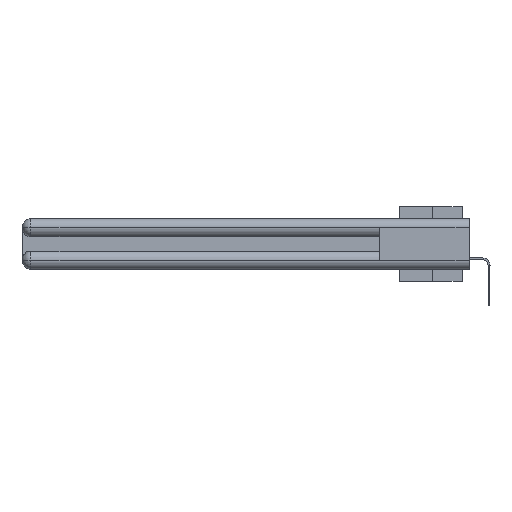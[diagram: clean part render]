
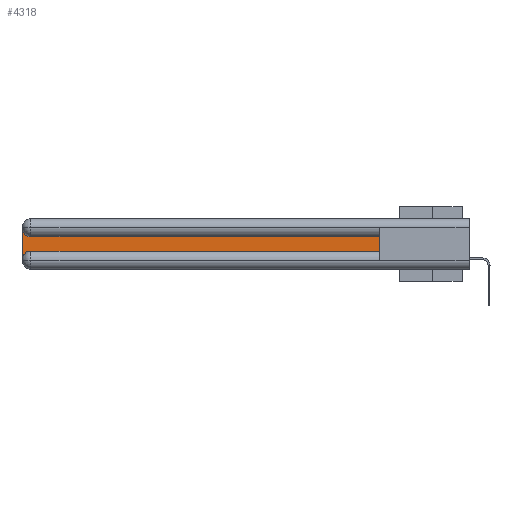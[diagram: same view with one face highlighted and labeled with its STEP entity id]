
A CAD part, left-side view. The second image highlights one B-rep face of the part: STEP entity #4318.
In plain terms, the highlighted planar face has unit normal (-1, 0, 0).
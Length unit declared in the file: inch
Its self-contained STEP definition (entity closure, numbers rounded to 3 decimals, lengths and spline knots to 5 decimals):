
#374 = CARTESIAN_POINT ( 'NONE',  ( 0.075, 2.94, -0.2775 ) ) ;
#1559 = LINE ( 'NONE', #11596, #24835 ) ;
#1977 = DIRECTION ( 'NONE',  ( 1., 0., 0. ) ) ;
#3443 = ORIENTED_EDGE ( 'NONE', *, *, #23956, .T. ) ;
#3686 = LINE ( 'NONE', #26589, #24172 ) ;
#4118 = VERTEX_POINT ( 'NONE', #25696 ) ;
#4223 = DIRECTION ( 'NONE',  ( 0., 0., -1. ) ) ;
#4318 = ADVANCED_FACE ( 'NONE', ( #4321 ), #12756, .F. ) ;
#4321 = FACE_OUTER_BOUND ( 'NONE', #5259, .T. ) ;
#4805 = DIRECTION ( 'NONE',  ( 1., 0., 0. ) ) ;
#5259 = EDGE_LOOP ( 'NONE', ( #17833, #15234, #28649, #16277, #9049, #3443 ) ) ;
#6048 = VERTEX_POINT ( 'NONE', #11331 ) ;
#7652 = VERTEX_POINT ( 'NONE', #13058 ) ;
#7880 = EDGE_CURVE ( 'NONE', #4118, #22042, #20739, .T. ) ;
#8345 = EDGE_CURVE ( 'NONE', #16306, #23847, #21772, .T. ) ;
#8831 = CARTESIAN_POINT ( 'NONE',  ( 0.075, 0.6, -0.2175 ) ) ;
#9049 = ORIENTED_EDGE ( 'NONE', *, *, #7880, .T. ) ;
#9163 = DIRECTION ( 'NONE',  ( 0., 0., -1. ) ) ;
#11331 = CARTESIAN_POINT ( 'NONE',  ( 0.075, 3., -0.2775 ) ) ;
#11596 = CARTESIAN_POINT ( 'NONE',  ( 0.075, 3., -0.2175 ) ) ;
#12555 = CARTESIAN_POINT ( 'NONE',  ( 0.075, 0.6, -0.2175 ) ) ;
#12756 = PLANE ( 'NONE',  #29003 ) ;
#13058 = CARTESIAN_POINT ( 'NONE',  ( 0.075, 0.6, -0.1225 ) ) ;
#13113 = CARTESIAN_POINT ( 'NONE',  ( 0.075, 2.94, -0.1225 ) ) ;
#13281 = CARTESIAN_POINT ( 'NONE',  ( 0.075, 2.94, -0.0625 ) ) ;
#14448 = DIRECTION ( 'NONE',  ( 0., -1., 0. ) ) ;
#14471 = DIRECTION ( 'NONE',  ( 0., 0., 1. ) ) ;
#15234 = ORIENTED_EDGE ( 'NONE', *, *, #8345, .T. ) ;
#15367 = EDGE_CURVE ( 'NONE', #6048, #4118, #16009, .T. ) ;
#16009 = CIRCLE ( 'NONE', #22250, 0.06 ) ;
#16148 = DIRECTION ( 'NONE',  ( 0., 0., -1. ) ) ;
#16277 = ORIENTED_EDGE ( 'NONE', *, *, #15367, .T. ) ;
#16306 = VERTEX_POINT ( 'NONE', #13113 ) ;
#16460 = AXIS2_PLACEMENT_3D ( 'NONE', #13281, #1977, #4223 ) ;
#16952 = CARTESIAN_POINT ( 'NONE',  ( 0.075, 0.6, -0.2175 ) ) ;
#17033 = DIRECTION ( 'NONE',  ( 0., 0., -1. ) ) ;
#17833 = ORIENTED_EDGE ( 'NONE', *, *, #27393, .T. ) ;
#19116 = EDGE_CURVE ( 'NONE', #23847, #6048, #1559, .T. ) ;
#20739 = LINE ( 'NONE', #12555, #27429 ) ;
#21772 = CIRCLE ( 'NONE', #16460, 0.06 ) ;
#21840 = CARTESIAN_POINT ( 'NONE',  ( 0.075, 3., -0.1225 ) ) ;
#22042 = VERTEX_POINT ( 'NONE', #8831 ) ;
#22250 = AXIS2_PLACEMENT_3D ( 'NONE', #374, #4805, #16148 ) ;
#22340 = DIRECTION ( 'NONE',  ( 0., 1., 0. ) ) ;
#23847 = VERTEX_POINT ( 'NONE', #25299 ) ;
#23867 = LINE ( 'NONE', #16952, #25255 ) ;
#23956 = EDGE_CURVE ( 'NONE', #22042, #7652, #23867, .T. ) ;
#24172 = VECTOR ( 'NONE', #22340, 39.37008 ) ;
#24835 = VECTOR ( 'NONE', #9163, 39.37008 ) ;
#25255 = VECTOR ( 'NONE', #14471, 39.37008 ) ;
#25299 = CARTESIAN_POINT ( 'NONE',  ( 0.075, 3., -0.0625 ) ) ;
#25696 = CARTESIAN_POINT ( 'NONE',  ( 0.075, 2.94, -0.2175 ) ) ;
#26471 = DIRECTION ( 'NONE',  ( 1., 0., 0. ) ) ;
#26589 = CARTESIAN_POINT ( 'NONE',  ( 0.075, 0.6, -0.1225 ) ) ;
#27393 = EDGE_CURVE ( 'NONE', #7652, #16306, #3686, .T. ) ;
#27429 = VECTOR ( 'NONE', #14448, 39.37008 ) ;
#28649 = ORIENTED_EDGE ( 'NONE', *, *, #19116, .T. ) ;
#29003 = AXIS2_PLACEMENT_3D ( 'NONE', #21840, #26471, #17033 ) ;
